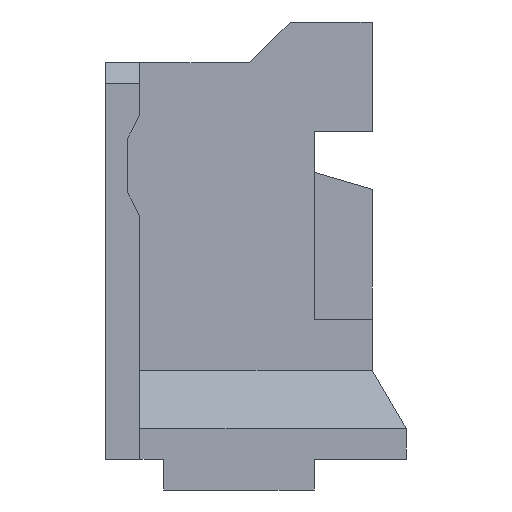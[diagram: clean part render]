
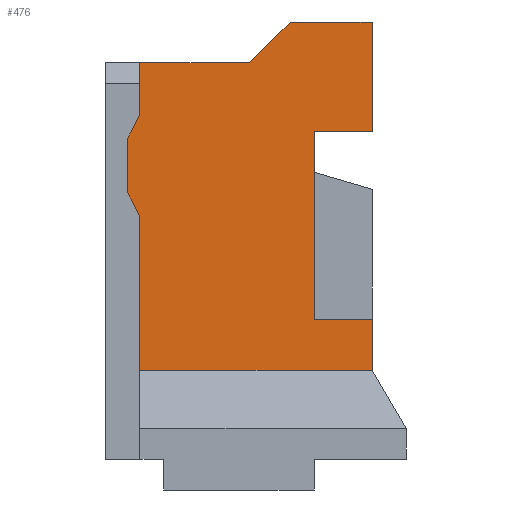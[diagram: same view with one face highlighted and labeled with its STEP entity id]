
A CAD part, left-side view. The second image highlights one B-rep face of the part: STEP entity #476.
In plain terms, the highlighted planar face has unit normal (-1, 0, 0).
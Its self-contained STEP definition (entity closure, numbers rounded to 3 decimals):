
#56 = VECTOR ( 'NONE', #2512, 1000. ) ;
#112 = VERTEX_POINT ( 'NONE', #4295 ) ;
#159 = LINE ( 'NONE', #3633, #56 ) ;
#160 = CARTESIAN_POINT ( 'NONE',  ( -1.25, 1.275, -2.25 ) ) ;
#167 = DIRECTION ( 'NONE',  ( 0., 0., 1. ) ) ;
#204 = CARTESIAN_POINT ( 'NONE',  ( -1.25, -1.1, 0.6 ) ) ;
#217 = LINE ( 'NONE', #4468, #1418 ) ;
#219 = ORIENTED_EDGE ( 'NONE', *, *, #3275, .F. ) ;
#437 = EDGE_CURVE ( 'NONE', #1903, #771, #3813, .T. ) ;
#476 = ADVANCED_FACE ( 'NONE', ( #533 ), #1884, .F. ) ;
#499 = ORIENTED_EDGE ( 'NONE', *, *, #1923, .F. ) ;
#533 = FACE_OUTER_BOUND ( 'NONE', #2321, .T. ) ;
#549 = VECTOR ( 'NONE', #2693, 1000. ) ;
#572 = EDGE_CURVE ( 'NONE', #2028, #4172, #1232, .T. ) ;
#596 = ORIENTED_EDGE ( 'NONE', *, *, #3788, .F. ) ;
#598 = VECTOR ( 'NONE', #167, 1000. ) ;
#661 = LINE ( 'NONE', #160, #549 ) ;
#719 = VERTEX_POINT ( 'NONE', #3604 ) ;
#720 = ORIENTED_EDGE ( 'NONE', *, *, #737, .F. ) ;
#737 = EDGE_CURVE ( 'NONE', #719, #1312, #1973, .T. ) ;
#771 = VERTEX_POINT ( 'NONE', #1495 ) ;
#789 = DIRECTION ( 'NONE',  ( 0., -0.707, 0.707 ) ) ;
#809 = CARTESIAN_POINT ( 'NONE',  ( -1.25, -2.3, -4.5 ) ) ;
#817 = VECTOR ( 'NONE', #2371, 1000. ) ;
#839 = CARTESIAN_POINT ( 'NONE',  ( -1.25, -1.45, -1. ) ) ;
#883 = EDGE_CURVE ( 'NONE', #3450, #112, #661, .T. ) ;
#950 = LINE ( 'NONE', #839, #4731 ) ;
#1042 = EDGE_CURVE ( 'NONE', #1301, #2844, #1352, .T. ) ;
#1180 = ORIENTED_EDGE ( 'NONE', *, *, #572, .F. ) ;
#1232 = LINE ( 'NONE', #3729, #3115 ) ;
#1249 = ORIENTED_EDGE ( 'NONE', *, *, #3498, .F. ) ;
#1283 = EDGE_CURVE ( 'NONE', #2844, #2028, #3010, .T. ) ;
#1284 = ORIENTED_EDGE ( 'NONE', *, *, #1283, .F. ) ;
#1301 = VERTEX_POINT ( 'NONE', #3239 ) ;
#1312 = VERTEX_POINT ( 'NONE', #2188 ) ;
#1344 = VECTOR ( 'NONE', #4042, 1000. ) ;
#1352 = LINE ( 'NONE', #2384, #598 ) ;
#1388 = VERTEX_POINT ( 'NONE', #809 ) ;
#1418 = VECTOR ( 'NONE', #2147, 1000. ) ;
#1419 = CARTESIAN_POINT ( 'NONE',  ( -1.25, 1.1, 0. ) ) ;
#1440 = CARTESIAN_POINT ( 'NONE',  ( -1.25, 0., 0. ) ) ;
#1450 = DIRECTION ( 'NONE',  ( 0., -1., 0. ) ) ;
#1495 = CARTESIAN_POINT ( 'NONE',  ( -1.25, -2.3, -1. ) ) ;
#1553 = CARTESIAN_POINT ( 'NONE',  ( -1.25, 1.275, -1.9 ) ) ;
#1594 = CARTESIAN_POINT ( 'NONE',  ( -1.25, 1.1, -2.25 ) ) ;
#1619 = DIRECTION ( 'NONE',  ( 0., 1., 0. ) ) ;
#1679 = ORIENTED_EDGE ( 'NONE', *, *, #4084, .F. ) ;
#1840 = CARTESIAN_POINT ( 'NONE',  ( -1.25, -2.3, 0.6 ) ) ;
#1871 = ORIENTED_EDGE ( 'NONE', *, *, #3097, .F. ) ;
#1884 = PLANE ( 'NONE',  #3092 ) ;
#1903 = VERTEX_POINT ( 'NONE', #3872 ) ;
#1923 = EDGE_CURVE ( 'NONE', #1388, #3379, #3507, .T. ) ;
#1973 = LINE ( 'NONE', #2860, #4711 ) ;
#1980 = VECTOR ( 'NONE', #2228, 1000. ) ;
#2028 = VERTEX_POINT ( 'NONE', #3956 ) ;
#2043 = ORIENTED_EDGE ( 'NONE', *, *, #4005, .F. ) ;
#2079 = CARTESIAN_POINT ( 'NONE',  ( -1.25, -3., -4.5 ) ) ;
#2147 = DIRECTION ( 'NONE',  ( 0., 0., 1. ) ) ;
#2188 = CARTESIAN_POINT ( 'NONE',  ( -1.25, -2.3, -3.75 ) ) ;
#2198 = VECTOR ( 'NONE', #1619, 1000. ) ;
#2207 = CARTESIAN_POINT ( 'NONE',  ( -1.25, -1.45, -1. ) ) ;
#2223 = VERTEX_POINT ( 'NONE', #2207 ) ;
#2228 = DIRECTION ( 'NONE',  ( 0., -1., 0. ) ) ;
#2321 = EDGE_LOOP ( 'NONE', ( #3183, #596, #2823, #1679, #219, #499, #1249, #720, #2043, #3164, #3764, #1871, #1180, #1284 ) ) ;
#2322 = EDGE_CURVE ( 'NONE', #771, #2223, #3686, .T. ) ;
#2370 = VERTEX_POINT ( 'NONE', #3811 ) ;
#2371 = DIRECTION ( 'NONE',  ( 0., -1., 0. ) ) ;
#2384 = CARTESIAN_POINT ( 'NONE',  ( -1.25, 1.1, -5.8 ) ) ;
#2435 = VECTOR ( 'NONE', #3607, 1000. ) ;
#2489 = CARTESIAN_POINT ( 'NONE',  ( -1.25, 1.1, -0.75 ) ) ;
#2512 = DIRECTION ( 'NONE',  ( 0., 0., -1. ) ) ;
#2630 = LINE ( 'NONE', #204, #817 ) ;
#2693 = DIRECTION ( 'NONE',  ( 0., 0., 1. ) ) ;
#2773 = CARTESIAN_POINT ( 'NONE',  ( -1.25, -1.1, 0.6 ) ) ;
#2823 = ORIENTED_EDGE ( 'NONE', *, *, #883, .F. ) ;
#2844 = VERTEX_POINT ( 'NONE', #3405 ) ;
#2860 = CARTESIAN_POINT ( 'NONE',  ( -1.25, 3.057, -3.75 ) ) ;
#3010 = LINE ( 'NONE', #1419, #1980 ) ;
#3092 = AXIS2_PLACEMENT_3D ( 'NONE', #1440, #3284, #4399 ) ;
#3097 = EDGE_CURVE ( 'NONE', #4172, #1903, #2630, .T. ) ;
#3115 = VECTOR ( 'NONE', #789, 1000. ) ;
#3163 = DIRECTION ( 'NONE',  ( 0., 1., 0. ) ) ;
#3164 = ORIENTED_EDGE ( 'NONE', *, *, #2322, .F. ) ;
#3183 = ORIENTED_EDGE ( 'NONE', *, *, #1042, .F. ) ;
#3239 = CARTESIAN_POINT ( 'NONE',  ( -1.25, 1.1, -0.75 ) ) ;
#3275 = EDGE_CURVE ( 'NONE', #3379, #2370, #217, .T. ) ;
#3284 = DIRECTION ( 'NONE',  ( 1., 0., 0. ) ) ;
#3379 = VERTEX_POINT ( 'NONE', #4349 ) ;
#3405 = CARTESIAN_POINT ( 'NONE',  ( -1.25, 1.1, 0. ) ) ;
#3423 = VECTOR ( 'NONE', #4128, 1000. ) ;
#3450 = VERTEX_POINT ( 'NONE', #1553 ) ;
#3498 = EDGE_CURVE ( 'NONE', #1312, #1388, #159, .T. ) ;
#3507 = LINE ( 'NONE', #2079, #3808 ) ;
#3604 = CARTESIAN_POINT ( 'NONE',  ( -1.25, -1.45, -3.75 ) ) ;
#3607 = DIRECTION ( 'NONE',  ( 0., -0.447, 0.894 ) ) ;
#3633 = CARTESIAN_POINT ( 'NONE',  ( -1.25, -2.3, -1.85 ) ) ;
#3647 = LINE ( 'NONE', #1594, #3423 ) ;
#3686 = LINE ( 'NONE', #4134, #2198 ) ;
#3729 = CARTESIAN_POINT ( 'NONE',  ( -1.25, -0.5, 0. ) ) ;
#3764 = ORIENTED_EDGE ( 'NONE', *, *, #437, .F. ) ;
#3788 = EDGE_CURVE ( 'NONE', #112, #1301, #4403, .T. ) ;
#3808 = VECTOR ( 'NONE', #3163, 1000. ) ;
#3811 = CARTESIAN_POINT ( 'NONE',  ( -1.25, 1.1, -2.25 ) ) ;
#3813 = LINE ( 'NONE', #1840, #1344 ) ;
#3872 = CARTESIAN_POINT ( 'NONE',  ( -1.25, -2.3, 0.6 ) ) ;
#3956 = CARTESIAN_POINT ( 'NONE',  ( -1.25, -0.5, 0. ) ) ;
#4005 = EDGE_CURVE ( 'NONE', #2223, #719, #950, .T. ) ;
#4042 = DIRECTION ( 'NONE',  ( 0., 0., -1. ) ) ;
#4084 = EDGE_CURVE ( 'NONE', #2370, #3450, #3647, .T. ) ;
#4128 = DIRECTION ( 'NONE',  ( 0., 0.447, 0.894 ) ) ;
#4134 = CARTESIAN_POINT ( 'NONE',  ( -1.25, -2.3, -1. ) ) ;
#4172 = VERTEX_POINT ( 'NONE', #2773 ) ;
#4295 = CARTESIAN_POINT ( 'NONE',  ( -1.25, 1.275, -1.1 ) ) ;
#4349 = CARTESIAN_POINT ( 'NONE',  ( -1.25, 1.1, -4.5 ) ) ;
#4399 = DIRECTION ( 'NONE',  ( 0., 0., -1. ) ) ;
#4403 = LINE ( 'NONE', #2489, #2435 ) ;
#4468 = CARTESIAN_POINT ( 'NONE',  ( -1.25, 1.1, -5.8 ) ) ;
#4504 = DIRECTION ( 'NONE',  ( 0., 0., -1. ) ) ;
#4711 = VECTOR ( 'NONE', #1450, 1000. ) ;
#4731 = VECTOR ( 'NONE', #4504, 1000. ) ;
